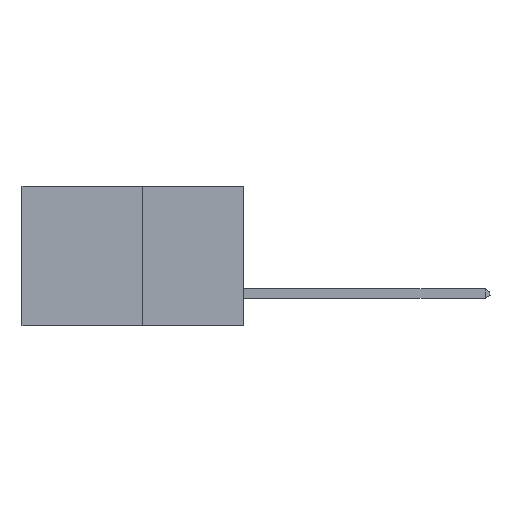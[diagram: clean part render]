
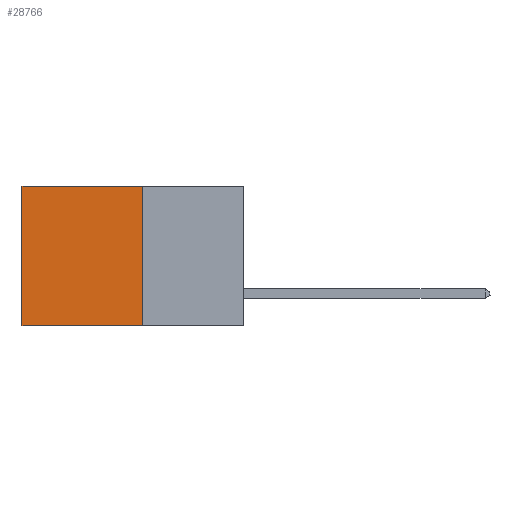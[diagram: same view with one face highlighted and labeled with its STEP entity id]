
A CAD part, left-side view. The second image highlights one B-rep face of the part: STEP entity #28766.
In plain terms, the highlighted planar face has unit normal (-1, 0, 0).
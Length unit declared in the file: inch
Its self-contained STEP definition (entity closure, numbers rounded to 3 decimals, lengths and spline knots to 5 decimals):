
#40 = CARTESIAN_POINT ( 'NONE',  ( 0.277, 0.59, -0.37 ) ) ;
#181 = VERTEX_POINT ( 'NONE', #3567 ) ;
#212 = EDGE_CURVE ( 'NONE', #27568, #30002, #17196, .T. ) ;
#257 = CARTESIAN_POINT ( 'NONE',  ( 0.277, 0.27, 0. ) ) ;
#2621 = LINE ( 'NONE', #27611, #27387 ) ;
#2809 = CARTESIAN_POINT ( 'NONE',  ( 0.277, 0.27, 0. ) ) ;
#3495 = EDGE_CURVE ( 'NONE', #30002, #4483, #2621, .T. ) ;
#3567 = CARTESIAN_POINT ( 'NONE',  ( 0.277, 0.59, 0. ) ) ;
#4419 = ORIENTED_EDGE ( 'NONE', *, *, #19248, .T. ) ;
#4483 = VERTEX_POINT ( 'NONE', #11805 ) ;
#4497 = DIRECTION ( 'NONE',  ( 0., 0., -1. ) ) ;
#4513 = ORIENTED_EDGE ( 'NONE', *, *, #27540, .T. ) ;
#5889 = DIRECTION ( 'NONE',  ( 0., 1., 0. ) ) ;
#6637 = ORIENTED_EDGE ( 'NONE', *, *, #3495, .F. ) ;
#9695 = DIRECTION ( 'NONE',  ( 0., 1., 0. ) ) ;
#11312 = VECTOR ( 'NONE', #9695, 39.37008 ) ;
#11705 = EDGE_LOOP ( 'NONE', ( #4419, #6637, #14851, #4513 ) ) ;
#11805 = CARTESIAN_POINT ( 'NONE',  ( 0.277, 0.59, -0.37 ) ) ;
#13368 = AXIS2_PLACEMENT_3D ( 'NONE', #16125, #18473, #4497 ) ;
#13519 = LINE ( 'NONE', #257, #11312 ) ;
#13834 = FACE_OUTER_BOUND ( 'NONE', #11705, .T. ) ;
#13938 = LINE ( 'NONE', #40, #26262 ) ;
#14851 = ORIENTED_EDGE ( 'NONE', *, *, #212, .F. ) ;
#16125 = CARTESIAN_POINT ( 'NONE',  ( 0.277, 0.27, -0.37 ) ) ;
#16349 = DIRECTION ( 'NONE',  ( 0., 0., -1. ) ) ;
#17196 = LINE ( 'NONE', #25870, #28040 ) ;
#18473 = DIRECTION ( 'NONE',  ( 1., 0., 0. ) ) ;
#19248 = EDGE_CURVE ( 'NONE', #181, #4483, #13938, .T. ) ;
#22748 = DIRECTION ( 'NONE',  ( 0., 0., -1. ) ) ;
#25844 = CARTESIAN_POINT ( 'NONE',  ( 0.277, 0.27, -0.37 ) ) ;
#25870 = CARTESIAN_POINT ( 'NONE',  ( 0.277, 0.27, -0.37 ) ) ;
#26262 = VECTOR ( 'NONE', #16349, 39.37008 ) ;
#27387 = VECTOR ( 'NONE', #5889, 39.37008 ) ;
#27540 = EDGE_CURVE ( 'NONE', #27568, #181, #13519, .T. ) ;
#27568 = VERTEX_POINT ( 'NONE', #2809 ) ;
#27611 = CARTESIAN_POINT ( 'NONE',  ( 0.277, 0.27, -0.37 ) ) ;
#28040 = VECTOR ( 'NONE', #22748, 39.37008 ) ;
#28766 = ADVANCED_FACE ( 'NONE', ( #13834 ), #30006, .F. ) ;
#30002 = VERTEX_POINT ( 'NONE', #25844 ) ;
#30006 = PLANE ( 'NONE',  #13368 ) ;
